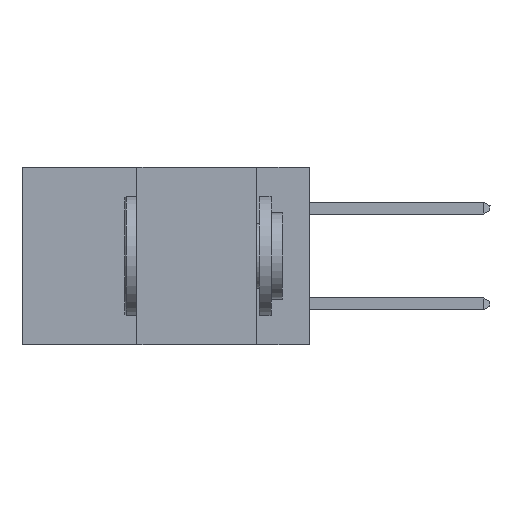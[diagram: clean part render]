
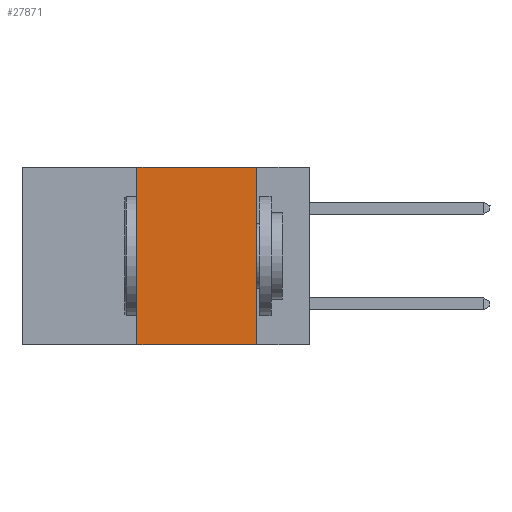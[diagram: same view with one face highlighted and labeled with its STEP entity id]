
A CAD part, left-side view. The second image highlights one B-rep face of the part: STEP entity #27871.
In plain terms, the highlighted planar face has unit normal (-1, 0, 0).
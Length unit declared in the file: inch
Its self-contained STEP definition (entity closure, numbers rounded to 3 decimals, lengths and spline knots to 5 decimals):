
#3550 = LINE ( 'NONE', #36565, #36579 ) ;
#4554 = EDGE_CURVE ( 'NONE', #14449, #39112, #26121, .T. ) ;
#4902 = CARTESIAN_POINT ( 'NONE',  ( 0., 0.36, -0.37 ) ) ;
#5612 = DIRECTION ( 'NONE',  ( 0., -1., 0. ) ) ;
#5696 = DIRECTION ( 'NONE',  ( 0., -1., 0. ) ) ;
#6502 = VECTOR ( 'NONE', #5696, 39.37008 ) ;
#8834 = VERTEX_POINT ( 'NONE', #39283 ) ;
#12580 = VERTEX_POINT ( 'NONE', #4902 ) ;
#12582 = LINE ( 'NONE', #14588, #37992 ) ;
#13168 = DIRECTION ( 'NONE',  ( 1., 0., 0. ) ) ;
#14449 = VERTEX_POINT ( 'NONE', #22777 ) ;
#14588 = CARTESIAN_POINT ( 'NONE',  ( 0., 0.6, -0.37 ) ) ;
#15710 = DIRECTION ( 'NONE',  ( 0., 0., 1. ) ) ;
#15967 = CARTESIAN_POINT ( 'NONE',  ( 0., 0.6, 0. ) ) ;
#16501 = DIRECTION ( 'NONE',  ( 0., 0., -1. ) ) ;
#18245 = DIRECTION ( 'NONE',  ( 0., 0., -1. ) ) ;
#18651 = ORIENTED_EDGE ( 'NONE', *, *, #19873, .T. ) ;
#18747 = ORIENTED_EDGE ( 'NONE', *, *, #29325, .F. ) ;
#19314 = EDGE_CURVE ( 'NONE', #39112, #8834, #3550, .T. ) ;
#19873 = EDGE_CURVE ( 'NONE', #12580, #8834, #12582, .T. ) ;
#20744 = CARTESIAN_POINT ( 'NONE',  ( 0., 0.6, 0. ) ) ;
#22777 = CARTESIAN_POINT ( 'NONE',  ( 0., 0.36, 0. ) ) ;
#22917 = CARTESIAN_POINT ( 'NONE',  ( 0., 0.11, 0. ) ) ;
#26121 = LINE ( 'NONE', #20744, #6502 ) ;
#26397 = ORIENTED_EDGE ( 'NONE', *, *, #19314, .F. ) ;
#27871 = ADVANCED_FACE ( 'NONE', ( #38853 ), #39145, .F. ) ;
#28886 = ORIENTED_EDGE ( 'NONE', *, *, #4554, .F. ) ;
#29325 = EDGE_CURVE ( 'NONE', #12580, #14449, #38294, .T. ) ;
#30121 = AXIS2_PLACEMENT_3D ( 'NONE', #15967, #13168, #16501 ) ;
#30939 = CARTESIAN_POINT ( 'NONE',  ( 0., 0.36, 0. ) ) ;
#31753 = EDGE_LOOP ( 'NONE', ( #26397, #28886, #18747, #18651 ) ) ;
#34434 = VECTOR ( 'NONE', #15710, 39.37008 ) ;
#36565 = CARTESIAN_POINT ( 'NONE',  ( 0., 0.11, 0. ) ) ;
#36579 = VECTOR ( 'NONE', #18245, 39.37008 ) ;
#37992 = VECTOR ( 'NONE', #5612, 39.37008 ) ;
#38294 = LINE ( 'NONE', #30939, #34434 ) ;
#38853 = FACE_OUTER_BOUND ( 'NONE', #31753, .T. ) ;
#39112 = VERTEX_POINT ( 'NONE', #22917 ) ;
#39145 = PLANE ( 'NONE',  #30121 ) ;
#39283 = CARTESIAN_POINT ( 'NONE',  ( 0., 0.11, -0.37 ) ) ;
